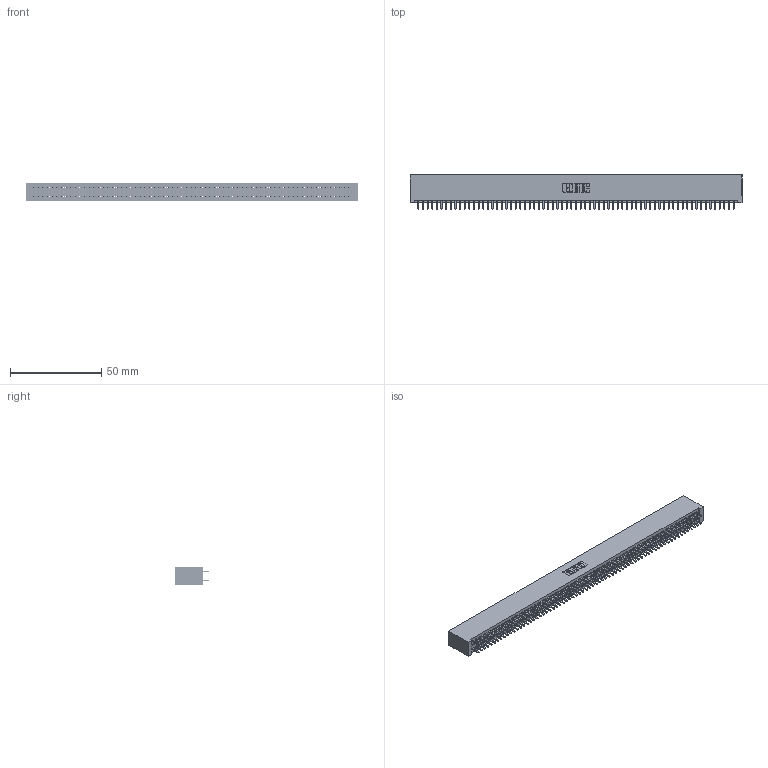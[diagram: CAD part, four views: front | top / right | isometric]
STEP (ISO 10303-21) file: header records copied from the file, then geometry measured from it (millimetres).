
FILE_DESCRIPTION (( 'STEP AP203' ), '1' );
FILE_NAME ('345-138-521-201.STEP', '2018-10-20T17:21:52', ( '' ), ( '' ), 'SwSTEP 2.0', 'SolidWorks 2016', '' );
FILE_SCHEMA (( 'CONFIG_CONTROL_DESIGN' ));
Length unit declared in the file: inch
Products named in the file (3): 345-292-001_345-293-121; 345 Part_No Mounting Lugs; 345-138-521-201
Assembly tree (139 placements, depth 2):
  345-138-521-201
    345 Part_No Mounting Lugs
    345-292-001_345-293-121  x138
Bounding box: 181.86 x 18.72 x 9.4 mm (x, y, z)
Volume: 18476.7 mm3; surface area: 27771.2 mm2
Topology: 139 solids, 139 shells, 7018 faces, 20879 edges, 13734 vertices
Faces by surface type: plane 4630, cylinder 2388
Entity records: 50245 total; most frequent: CARTESIAN_POINT 8396, ORIENTED_EDGE 8330, DIRECTION 7365, EDGE_CURVE 4165, LINE 3765, VECTOR 3765, VERTEX_POINT 2774, AXIS2_PLACEMENT_3D 1800
